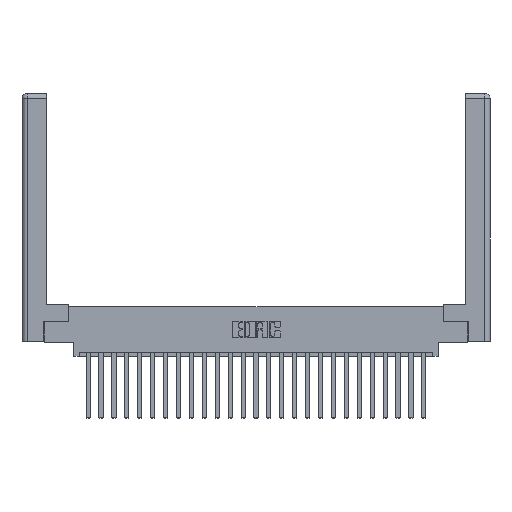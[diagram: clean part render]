
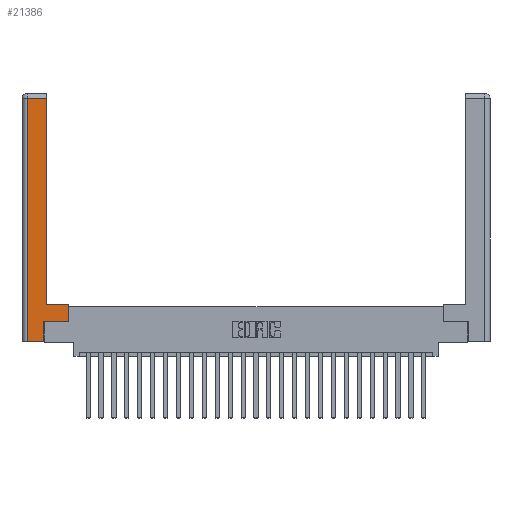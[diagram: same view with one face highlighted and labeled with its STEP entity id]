
A CAD part, top view. The second image highlights one B-rep face of the part: STEP entity #21386.
In plain terms, the highlighted planar face has unit normal (0, 0, 1).
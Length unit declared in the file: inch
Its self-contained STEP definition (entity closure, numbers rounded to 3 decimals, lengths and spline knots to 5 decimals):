
#446 = CARTESIAN_POINT ( 'NONE',  ( 0.565, 0.245, 0. ) ) ;
#918 = EDGE_CURVE ( 'NONE', #7865, #1435, #11578, .T. ) ;
#1121 = EDGE_CURVE ( 'NONE', #15145, #7865, #4780, .T. ) ;
#1435 = VERTEX_POINT ( 'NONE', #14337 ) ;
#1654 = CARTESIAN_POINT ( 'NONE',  ( 0.0615, 0., 0. ) ) ;
#2071 = CARTESIAN_POINT ( 'NONE',  ( 0.565, 0.245, 0. ) ) ;
#2768 = EDGE_CURVE ( 'NONE', #5003, #14522, #9051, .T. ) ;
#2810 = AXIS2_PLACEMENT_3D ( 'NONE', #23156, #7206, #11365 ) ;
#3023 = ORIENTED_EDGE ( 'NONE', *, *, #17572, .T. ) ;
#3413 = PLANE ( 'NONE',  #2810 ) ;
#3946 = FACE_OUTER_BOUND ( 'NONE', #6834, .T. ) ;
#4219 = EDGE_CURVE ( 'NONE', #10486, #15145, #11776, .T. ) ;
#4730 = ORIENTED_EDGE ( 'NONE', *, *, #4219, .T. ) ;
#4780 = LINE ( 'NONE', #13246, #13091 ) ;
#4954 = ORIENTED_EDGE ( 'NONE', *, *, #1121, .T. ) ;
#5003 = VERTEX_POINT ( 'NONE', #11686 ) ;
#5687 = VECTOR ( 'NONE', #17913, 39.37008 ) ;
#6309 = VECTOR ( 'NONE', #25404, 39.37008 ) ;
#6825 = CARTESIAN_POINT ( 'NONE',  ( 0.295, 0.45, 0. ) ) ;
#6834 = EDGE_LOOP ( 'NONE', ( #4730, #4954, #10645, #8637, #3023, #16081, #23717, #13457 ) ) ;
#7206 = DIRECTION ( 'NONE',  ( 0., 0., -1. ) ) ;
#7323 = DIRECTION ( 'NONE',  ( 0., 1., 0. ) ) ;
#7865 = VERTEX_POINT ( 'NONE', #13761 ) ;
#8637 = ORIENTED_EDGE ( 'NONE', *, *, #10093, .T. ) ;
#8747 = LINE ( 'NONE', #19718, #9984 ) ;
#9051 = LINE ( 'NONE', #446, #5687 ) ;
#9391 = LINE ( 'NONE', #13400, #15606 ) ;
#9984 = VECTOR ( 'NONE', #20055, 39.37008 ) ;
#10093 = EDGE_CURVE ( 'NONE', #1435, #15412, #8747, .T. ) ;
#10486 = VERTEX_POINT ( 'NONE', #6825 ) ;
#10645 = ORIENTED_EDGE ( 'NONE', *, *, #918, .T. ) ;
#11365 = DIRECTION ( 'NONE',  ( -1., 0., 0. ) ) ;
#11578 = LINE ( 'NONE', #1654, #6309 ) ;
#11686 = CARTESIAN_POINT ( 'NONE',  ( 0.265, 0.245, 0. ) ) ;
#11776 = LINE ( 'NONE', #24983, #23793 ) ;
#11939 = VECTOR ( 'NONE', #22955, 39.37008 ) ;
#12844 = EDGE_CURVE ( 'NONE', #21372, #10486, #9391, .T. ) ;
#13091 = VECTOR ( 'NONE', #13424, 39.37008 ) ;
#13246 = CARTESIAN_POINT ( 'NONE',  ( 0.0615, 2.94, 0. ) ) ;
#13400 = CARTESIAN_POINT ( 'NONE',  ( 0.295, 0.45, 0. ) ) ;
#13424 = DIRECTION ( 'NONE',  ( -1., 0., 0. ) ) ;
#13457 = ORIENTED_EDGE ( 'NONE', *, *, #12844, .T. ) ;
#13761 = CARTESIAN_POINT ( 'NONE',  ( 0.0615, 2.94, 0. ) ) ;
#13783 = LINE ( 'NONE', #15265, #11939 ) ;
#14337 = CARTESIAN_POINT ( 'NONE',  ( 0.0615, 0., 0. ) ) ;
#14389 = LINE ( 'NONE', #24172, #22745 ) ;
#14409 = DIRECTION ( 'NONE',  ( 0., 1., 0. ) ) ;
#14522 = VERTEX_POINT ( 'NONE', #2071 ) ;
#15145 = VERTEX_POINT ( 'NONE', #19540 ) ;
#15265 = CARTESIAN_POINT ( 'NONE',  ( 0.565, 0.45, 0. ) ) ;
#15412 = VERTEX_POINT ( 'NONE', #17678 ) ;
#15606 = VECTOR ( 'NONE', #25428, 39.37008 ) ;
#16081 = ORIENTED_EDGE ( 'NONE', *, *, #2768, .T. ) ;
#17572 = EDGE_CURVE ( 'NONE', #15412, #5003, #14389, .T. ) ;
#17678 = CARTESIAN_POINT ( 'NONE',  ( 0.265, 0., 0. ) ) ;
#17913 = DIRECTION ( 'NONE',  ( 1., 0., 0. ) ) ;
#19087 = CARTESIAN_POINT ( 'NONE',  ( 0.565, 0.45, 0. ) ) ;
#19540 = CARTESIAN_POINT ( 'NONE',  ( 0.295, 2.94, 0. ) ) ;
#19718 = CARTESIAN_POINT ( 'NONE',  ( 0.265, 0., 0. ) ) ;
#20055 = DIRECTION ( 'NONE',  ( 1., 0., 0. ) ) ;
#21372 = VERTEX_POINT ( 'NONE', #19087 ) ;
#21386 = ADVANCED_FACE ( 'NONE', ( #3946 ), #3413, .F. ) ;
#22745 = VECTOR ( 'NONE', #14409, 39.37008 ) ;
#22955 = DIRECTION ( 'NONE',  ( 0., 1., 0. ) ) ;
#23156 = CARTESIAN_POINT ( 'NONE',  ( 0., 0., 0. ) ) ;
#23717 = ORIENTED_EDGE ( 'NONE', *, *, #25163, .T. ) ;
#23793 = VECTOR ( 'NONE', #7323, 39.37008 ) ;
#24172 = CARTESIAN_POINT ( 'NONE',  ( 0.265, 0.245, 0. ) ) ;
#24983 = CARTESIAN_POINT ( 'NONE',  ( 0.295, 3., 0. ) ) ;
#25163 = EDGE_CURVE ( 'NONE', #14522, #21372, #13783, .T. ) ;
#25404 = DIRECTION ( 'NONE',  ( 0., -1., 0. ) ) ;
#25428 = DIRECTION ( 'NONE',  ( -1., 0., 0. ) ) ;
